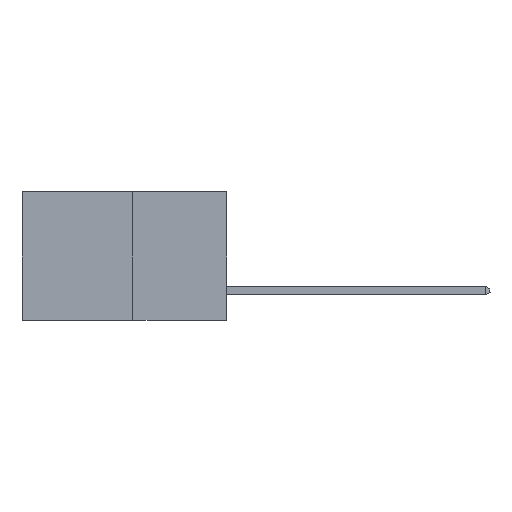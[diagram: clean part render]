
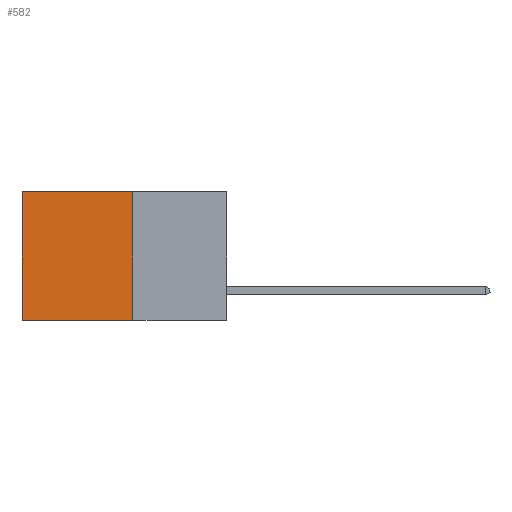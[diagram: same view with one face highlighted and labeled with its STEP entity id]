
A CAD part, left-side view. The second image highlights one B-rep face of the part: STEP entity #582.
In plain terms, the highlighted planar face has unit normal (-1, 0, 0).
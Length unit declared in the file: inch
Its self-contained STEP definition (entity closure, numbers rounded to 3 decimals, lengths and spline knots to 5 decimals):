
#133 = DIRECTION ( 'NONE',  ( 1., 0., 0. ) ) ;
#137 = PLANE ( 'NONE',  #13830 ) ;
#582 = ADVANCED_FACE ( 'NONE', ( #14439 ), #137, .F. ) ;
#963 = VERTEX_POINT ( 'NONE', #10377 ) ;
#1576 = CARTESIAN_POINT ( 'NONE',  ( 0.277, 0.27, 0. ) ) ;
#2133 = ORIENTED_EDGE ( 'NONE', *, *, #8987, .F. ) ;
#2539 = ORIENTED_EDGE ( 'NONE', *, *, #6348, .F. ) ;
#2618 = CARTESIAN_POINT ( 'NONE',  ( 0.277, 0.27, 0. ) ) ;
#2696 = LINE ( 'NONE', #4843, #8518 ) ;
#3279 = EDGE_LOOP ( 'NONE', ( #9469, #2539, #2133, #7653 ) ) ;
#4652 = CARTESIAN_POINT ( 'NONE',  ( 0.277, 0.27, -0.37 ) ) ;
#4843 = CARTESIAN_POINT ( 'NONE',  ( 0.277, 0.59, -0.37 ) ) ;
#4865 = DIRECTION ( 'NONE',  ( 0., 1., 0. ) ) ;
#5211 = CARTESIAN_POINT ( 'NONE',  ( 0.277, 0.59, 0. ) ) ;
#6033 = DIRECTION ( 'NONE',  ( 0., 0., -1. ) ) ;
#6323 = CARTESIAN_POINT ( 'NONE',  ( 0.277, 0.59, -0.37 ) ) ;
#6335 = VERTEX_POINT ( 'NONE', #5211 ) ;
#6348 = EDGE_CURVE ( 'NONE', #963, #7395, #10212, .T. ) ;
#7395 = VERTEX_POINT ( 'NONE', #6323 ) ;
#7653 = ORIENTED_EDGE ( 'NONE', *, *, #11476, .T. ) ;
#8207 = CARTESIAN_POINT ( 'NONE',  ( 0.277, 0.27, -0.37 ) ) ;
#8518 = VECTOR ( 'NONE', #6033, 39.37008 ) ;
#8987 = EDGE_CURVE ( 'NONE', #11389, #963, #10126, .T. ) ;
#9428 = DIRECTION ( 'NONE',  ( 0., 0., -1. ) ) ;
#9469 = ORIENTED_EDGE ( 'NONE', *, *, #11271, .T. ) ;
#9473 = LINE ( 'NONE', #1576, #13822 ) ;
#9678 = DIRECTION ( 'NONE',  ( 0., 1., 0. ) ) ;
#10126 = LINE ( 'NONE', #10393, #12640 ) ;
#10212 = LINE ( 'NONE', #8207, #12719 ) ;
#10377 = CARTESIAN_POINT ( 'NONE',  ( 0.277, 0.27, -0.37 ) ) ;
#10393 = CARTESIAN_POINT ( 'NONE',  ( 0.277, 0.27, -0.37 ) ) ;
#11271 = EDGE_CURVE ( 'NONE', #6335, #7395, #2696, .T. ) ;
#11389 = VERTEX_POINT ( 'NONE', #2618 ) ;
#11476 = EDGE_CURVE ( 'NONE', #11389, #6335, #9473, .T. ) ;
#11486 = DIRECTION ( 'NONE',  ( 0., 0., -1. ) ) ;
#12640 = VECTOR ( 'NONE', #11486, 39.37008 ) ;
#12719 = VECTOR ( 'NONE', #4865, 39.37008 ) ;
#13822 = VECTOR ( 'NONE', #9678, 39.37008 ) ;
#13830 = AXIS2_PLACEMENT_3D ( 'NONE', #4652, #133, #9428 ) ;
#14439 = FACE_OUTER_BOUND ( 'NONE', #3279, .T. ) ;
